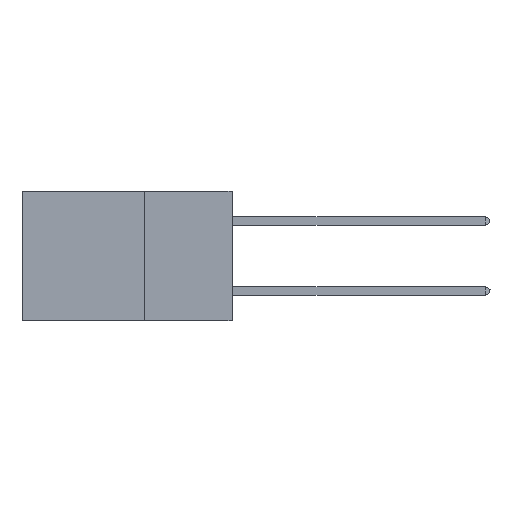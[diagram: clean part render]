
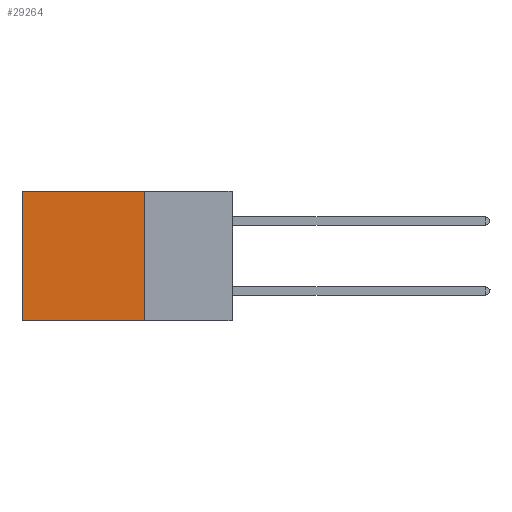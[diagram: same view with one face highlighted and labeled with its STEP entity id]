
A CAD part, left-side view. The second image highlights one B-rep face of the part: STEP entity #29264.
In plain terms, the highlighted planar face has unit normal (-1, 0, 0).
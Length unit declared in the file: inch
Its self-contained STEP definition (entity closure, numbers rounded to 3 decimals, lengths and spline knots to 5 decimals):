
#1365 = CARTESIAN_POINT ( 'NONE',  ( 0.2875, 0.6, -0.37 ) ) ;
#2597 = DIRECTION ( 'NONE',  ( 0., 1., 0. ) ) ;
#4209 = DIRECTION ( 'NONE',  ( 0., 0., -1. ) ) ;
#4638 = CARTESIAN_POINT ( 'NONE',  ( 0.2875, 0.25, -0.37 ) ) ;
#5987 = VERTEX_POINT ( 'NONE', #35546 ) ;
#7360 = EDGE_CURVE ( 'NONE', #12322, #5987, #8943, .T. ) ;
#8943 = LINE ( 'NONE', #24644, #19110 ) ;
#10465 = CARTESIAN_POINT ( 'NONE',  ( 0.2875, 0.6, 0. ) ) ;
#11216 = PLANE ( 'NONE',  #29507 ) ;
#12322 = VERTEX_POINT ( 'NONE', #33775 ) ;
#13311 = VERTEX_POINT ( 'NONE', #1365 ) ;
#13915 = DIRECTION ( 'NONE',  ( 1., 0., 0. ) ) ;
#14001 = DIRECTION ( 'NONE',  ( 0., 1., 0. ) ) ;
#14942 = EDGE_CURVE ( 'NONE', #5987, #13311, #39414, .T. ) ;
#16366 = VECTOR ( 'NONE', #4209, 39.37008 ) ;
#16887 = CARTESIAN_POINT ( 'NONE',  ( 0.2875, 0.25, 0. ) ) ;
#19005 = FACE_OUTER_BOUND ( 'NONE', #24513, .T. ) ;
#19110 = VECTOR ( 'NONE', #19963, 39.37008 ) ;
#19963 = DIRECTION ( 'NONE',  ( 0., 0., -1. ) ) ;
#23296 = EDGE_CURVE ( 'NONE', #24131, #13311, #29465, .T. ) ;
#24131 = VERTEX_POINT ( 'NONE', #27395 ) ;
#24175 = EDGE_CURVE ( 'NONE', #12322, #24131, #34176, .T. ) ;
#24513 = EDGE_LOOP ( 'NONE', ( #25876, #35592, #39708, #24619 ) ) ;
#24619 = ORIENTED_EDGE ( 'NONE', *, *, #24175, .T. ) ;
#24644 = CARTESIAN_POINT ( 'NONE',  ( 0.2875, 0.25, 0. ) ) ;
#25876 = ORIENTED_EDGE ( 'NONE', *, *, #23296, .T. ) ;
#27395 = CARTESIAN_POINT ( 'NONE',  ( 0.2875, 0.6, 0. ) ) ;
#29264 = ADVANCED_FACE ( 'NONE', ( #19005 ), #11216, .F. ) ;
#29465 = LINE ( 'NONE', #10465, #16366 ) ;
#29507 = AXIS2_PLACEMENT_3D ( 'NONE', #16887, #13915, #35773 ) ;
#31028 = CARTESIAN_POINT ( 'NONE',  ( 0.2875, 0.25, 0. ) ) ;
#33229 = VECTOR ( 'NONE', #2597, 39.37008 ) ;
#33775 = CARTESIAN_POINT ( 'NONE',  ( 0.2875, 0.25, 0. ) ) ;
#34176 = LINE ( 'NONE', #31028, #33229 ) ;
#35546 = CARTESIAN_POINT ( 'NONE',  ( 0.2875, 0.25, -0.37 ) ) ;
#35592 = ORIENTED_EDGE ( 'NONE', *, *, #14942, .F. ) ;
#35773 = DIRECTION ( 'NONE',  ( 0., 0., -1. ) ) ;
#35994 = VECTOR ( 'NONE', #14001, 39.37008 ) ;
#39414 = LINE ( 'NONE', #4638, #35994 ) ;
#39708 = ORIENTED_EDGE ( 'NONE', *, *, #7360, .F. ) ;
